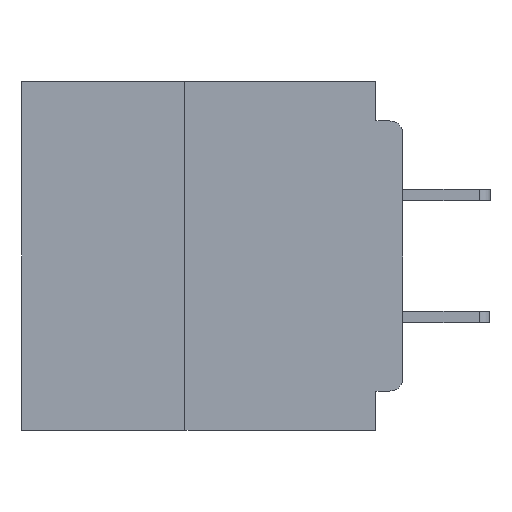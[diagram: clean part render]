
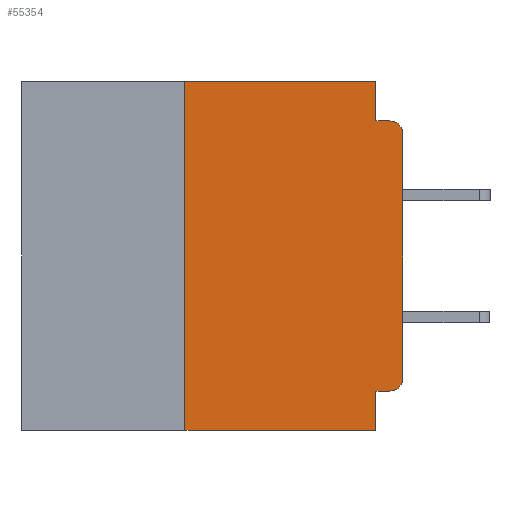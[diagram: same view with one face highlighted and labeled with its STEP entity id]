
A CAD part, left-side view. The second image highlights one B-rep face of the part: STEP entity #55354.
In plain terms, the highlighted planar face has unit normal (-1, 0, 0).
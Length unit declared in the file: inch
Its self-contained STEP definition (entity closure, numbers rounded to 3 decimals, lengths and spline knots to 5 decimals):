
#762 = VERTEX_POINT ( 'NONE', #38800 ) ;
#2245 = VERTEX_POINT ( 'NONE', #25818 ) ;
#2925 = ORIENTED_EDGE ( 'NONE', *, *, #23314, .T. ) ;
#3666 = DIRECTION ( 'NONE',  ( 0., 0., -1. ) ) ;
#4450 = ORIENTED_EDGE ( 'NONE', *, *, #23388, .F. ) ;
#5830 = VECTOR ( 'NONE', #37787, 39.37008 ) ;
#5876 = CARTESIAN_POINT ( 'NONE',  ( 0., 0.031, -0.4 ) ) ;
#6106 = CARTESIAN_POINT ( 'NONE',  ( 0., 0.25, -0.4 ) ) ;
#6174 = CIRCLE ( 'NONE', #43319, 0.015 ) ;
#6478 = CARTESIAN_POINT ( 'NONE',  ( 0., 0.437, 0. ) ) ;
#7277 = VECTOR ( 'NONE', #37539, 39.37008 ) ;
#7873 = ORIENTED_EDGE ( 'NONE', *, *, #27643, .T. ) ;
#8468 = VECTOR ( 'NONE', #22965, 39.37008 ) ;
#8575 = CARTESIAN_POINT ( 'NONE',  ( 0., 0., -0.34 ) ) ;
#9126 = EDGE_CURVE ( 'NONE', #35226, #11488, #6174, .T. ) ;
#9702 = DIRECTION ( 'NONE',  ( -1., 0., 0. ) ) ;
#10199 = PLANE ( 'NONE',  #31264 ) ;
#10799 = VECTOR ( 'NONE', #38132, 39.37008 ) ;
#11253 = ORIENTED_EDGE ( 'NONE', *, *, #53380, .T. ) ;
#11488 = VERTEX_POINT ( 'NONE', #8575 ) ;
#11806 = ORIENTED_EDGE ( 'NONE', *, *, #9126, .T. ) ;
#11810 = EDGE_CURVE ( 'NONE', #19180, #29214, #19266, .T. ) ;
#12124 = ORIENTED_EDGE ( 'NONE', *, *, #49586, .F. ) ;
#12704 = ORIENTED_EDGE ( 'NONE', *, *, #11810, .F. ) ;
#12705 = LINE ( 'NONE', #22773, #35394 ) ;
#15216 = CARTESIAN_POINT ( 'NONE',  ( 0., 0.25, -0.4 ) ) ;
#15637 = LINE ( 'NONE', #24526, #50181 ) ;
#15930 = ORIENTED_EDGE ( 'NONE', *, *, #27691, .F. ) ;
#17486 = LINE ( 'NONE', #22468, #40158 ) ;
#17516 = CARTESIAN_POINT ( 'NONE',  ( 0., 0.437, -0.4 ) ) ;
#17531 = EDGE_LOOP ( 'NONE', ( #7873, #11253, #15930, #4450, #12124, #12704, #2925, #29356, #27014, #11806 ) ) ;
#19180 = VERTEX_POINT ( 'NONE', #6106 ) ;
#19266 = LINE ( 'NONE', #15216, #5830 ) ;
#19268 = LINE ( 'NONE', #5876, #7277 ) ;
#19274 = DIRECTION ( 'NONE',  ( 0., 0., -1. ) ) ;
#20280 = CARTESIAN_POINT ( 'NONE',  ( 0., 0.031, 0. ) ) ;
#20744 = VERTEX_POINT ( 'NONE', #33369 ) ;
#21024 = CARTESIAN_POINT ( 'NONE',  ( 0., 0.031, -0.045 ) ) ;
#21401 = EDGE_CURVE ( 'NONE', #35226, #20744, #15637, .T. ) ;
#22468 = CARTESIAN_POINT ( 'NONE',  ( 0., 0.031, 0. ) ) ;
#22773 = CARTESIAN_POINT ( 'NONE',  ( 0., 0., 0. ) ) ;
#22815 = LINE ( 'NONE', #6478, #10799 ) ;
#22965 = DIRECTION ( 'NONE',  ( 0., -1., 0. ) ) ;
#23314 = EDGE_CURVE ( 'NONE', #19180, #2245, #54797, .T. ) ;
#23388 = EDGE_CURVE ( 'NONE', #42084, #55645, #17486, .T. ) ;
#24526 = CARTESIAN_POINT ( 'NONE',  ( 0., 0., -0.355 ) ) ;
#25818 = CARTESIAN_POINT ( 'NONE',  ( 0., 0.031, -0.4 ) ) ;
#27014 = ORIENTED_EDGE ( 'NONE', *, *, #21401, .F. ) ;
#27643 = EDGE_CURVE ( 'NONE', #11488, #762, #12705, .T. ) ;
#27691 = EDGE_CURVE ( 'NONE', #55645, #33836, #56309, .T. ) ;
#29214 = VERTEX_POINT ( 'NONE', #29272 ) ;
#29272 = CARTESIAN_POINT ( 'NONE',  ( 0., 0.25, 0. ) ) ;
#29356 = ORIENTED_EDGE ( 'NONE', *, *, #32208, .F. ) ;
#30836 = DIRECTION ( 'NONE',  ( -1., 0., 0. ) ) ;
#31264 = AXIS2_PLACEMENT_3D ( 'NONE', #41840, #46338, #19274 ) ;
#32208 = EDGE_CURVE ( 'NONE', #20744, #2245, #19268, .T. ) ;
#32279 = AXIS2_PLACEMENT_3D ( 'NONE', #36828, #9702, #41332 ) ;
#33369 = CARTESIAN_POINT ( 'NONE',  ( 0., 0.031, -0.355 ) ) ;
#33836 = VERTEX_POINT ( 'NONE', #53590 ) ;
#35226 = VERTEX_POINT ( 'NONE', #55155 ) ;
#35394 = VECTOR ( 'NONE', #54227, 39.37008 ) ;
#36828 = CARTESIAN_POINT ( 'NONE',  ( 0., 0.015, -0.06 ) ) ;
#37539 = DIRECTION ( 'NONE',  ( 0., 0., -1. ) ) ;
#37787 = DIRECTION ( 'NONE',  ( 0., 0., 1. ) ) ;
#38132 = DIRECTION ( 'NONE',  ( 0., -1., 0. ) ) ;
#38800 = CARTESIAN_POINT ( 'NONE',  ( 0., 0., -0.06 ) ) ;
#40158 = VECTOR ( 'NONE', #40476, 39.37008 ) ;
#40476 = DIRECTION ( 'NONE',  ( 0., 0., -1. ) ) ;
#41332 = DIRECTION ( 'NONE',  ( 0., 0., -1. ) ) ;
#41840 = CARTESIAN_POINT ( 'NONE',  ( 0., 0.437, 0. ) ) ;
#42084 = VERTEX_POINT ( 'NONE', #20280 ) ;
#43319 = AXIS2_PLACEMENT_3D ( 'NONE', #57589, #30836, #3666 ) ;
#46338 = DIRECTION ( 'NONE',  ( 1., 0., 0. ) ) ;
#49091 = DIRECTION ( 'NONE',  ( 0., -1., 0. ) ) ;
#49586 = EDGE_CURVE ( 'NONE', #29214, #42084, #22815, .T. ) ;
#49716 = FACE_OUTER_BOUND ( 'NONE', #17531, .T. ) ;
#49949 = CARTESIAN_POINT ( 'NONE',  ( 0., 0., -0.045 ) ) ;
#50181 = VECTOR ( 'NONE', #55935, 39.37008 ) ;
#53380 = EDGE_CURVE ( 'NONE', #762, #33836, #58239, .T. ) ;
#53590 = CARTESIAN_POINT ( 'NONE',  ( 0., 0.015, -0.045 ) ) ;
#54227 = DIRECTION ( 'NONE',  ( 0., 0., 1. ) ) ;
#54797 = LINE ( 'NONE', #17516, #56191 ) ;
#55155 = CARTESIAN_POINT ( 'NONE',  ( 0., 0.015, -0.355 ) ) ;
#55354 = ADVANCED_FACE ( 'NONE', ( #49716 ), #10199, .F. ) ;
#55645 = VERTEX_POINT ( 'NONE', #21024 ) ;
#55935 = DIRECTION ( 'NONE',  ( 0., 1., 0. ) ) ;
#56191 = VECTOR ( 'NONE', #49091, 39.37008 ) ;
#56309 = LINE ( 'NONE', #49949, #8468 ) ;
#57589 = CARTESIAN_POINT ( 'NONE',  ( 0., 0.015, -0.34 ) ) ;
#58239 = CIRCLE ( 'NONE', #32279, 0.015 ) ;
